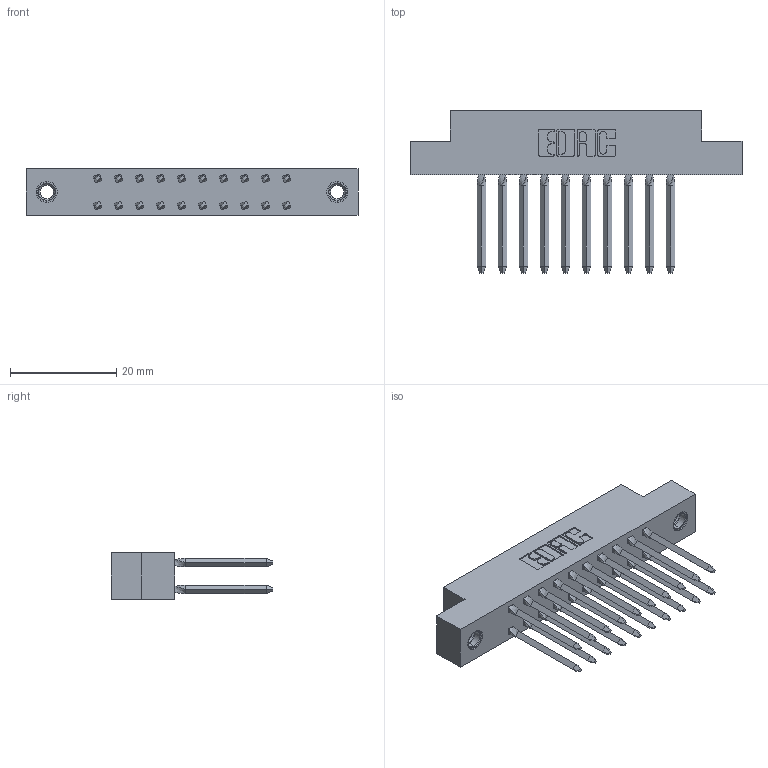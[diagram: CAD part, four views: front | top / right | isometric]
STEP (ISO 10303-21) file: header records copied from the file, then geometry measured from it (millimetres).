
FILE_DESCRIPTION (( 'STEP AP203' ), '1' );
FILE_NAME ('338-020-541-207.STEP', '2020-03-24T17:33:24', ( '' ), ( '' ), 'SwSTEP 2.0', 'SolidWorks 2016', '' );
FILE_SCHEMA (( 'CONFIG_CONTROL_DESIGN' ));
Length unit declared in the file: inch
Products named in the file (4): 338-290-001_541; 345-250-001_345-250-005-103; 338-020-541-207; 338-210-001_338-210-010-004
Assembly tree (23 placements, depth 2):
  338-020-541-207
    338-210-001_338-210-010-004
    338-290-001_541  x20
    345-250-001_345-250-005-103  x2
Bounding box: 62.64 x 30.56 x 8.71 mm (x, y, z)
Volume: 4664.4 mm3; surface area: 7949.8 mm2
Topology: 23 solids, 23 shells, 1494 faces, 3987 edges, 2530 vertices
Faces by surface type: plane 1022, cylinder 376, bspline 80, cone 12, torus 4
Entity records: 24109 total; most frequent: CARTESIAN_POINT 4803, ORIENTED_EDGE 3960, DIRECTION 3721, EDGE_CURVE 1980, LINE 1429, VECTOR 1429, VERTEX_POINT 1284, AXIS2_PLACEMENT_3D 1146
